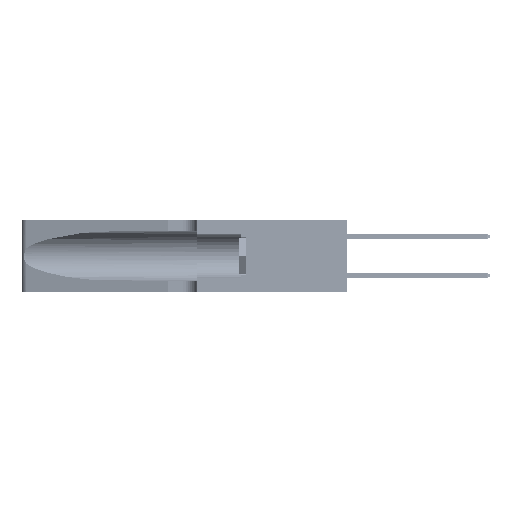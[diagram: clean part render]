
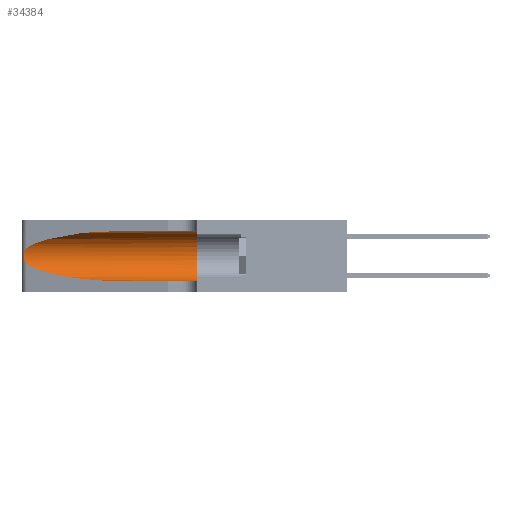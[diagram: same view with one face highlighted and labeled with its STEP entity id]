
A CAD part, left-side view. The second image highlights one B-rep face of the part: STEP entity #34384.
In plain terms, the highlighted cylindrical face has radius 3.308 mm (diameter 6.617 mm), a partial arc.
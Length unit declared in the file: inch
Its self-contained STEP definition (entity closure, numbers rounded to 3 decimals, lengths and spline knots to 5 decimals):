
#969 = VERTEX_POINT ( 'NONE', #30468 ) ;
#2251 = EDGE_CURVE ( 'NONE', #35612, #40799, #40156, .T. ) ;
#2321 = VECTOR ( 'NONE', #39115, 39.37008 ) ;
#2410 = CARTESIAN_POINT ( 'NONE',  ( 0.25555, 1.22993, 0.14849 ) ) ;
#3430 = EDGE_LOOP ( 'NONE', ( #4043, #3513, #14222, #49660, #28067, #21166 ) ) ;
#3513 = ORIENTED_EDGE ( 'NONE', *, *, #25475, .T. ) ;
#3804 = CARTESIAN_POINT ( 'NONE',  ( 0.1305, 1.61858, 0.185 ) ) ;
#3855 =( BOUNDED_CURVE ( )  B_SPLINE_CURVE ( 3, ( #22449, #6502, #34517, #10548 ),
 .UNSPECIFIED., .F., .F. ) 
 B_SPLINE_CURVE_WITH_KNOTS ( ( 4, 4 ),
 ( 3.44316, 4.71239 ),
 .UNSPECIFIED. ) 
 CURVE ( )  GEOMETRIC_REPRESENTATION_ITEM ( )  RATIONAL_B_SPLINE_CURVE ( ( 1., 0.87, 0.87, 1. ) ) 
 REPRESENTATION_ITEM ( '' )  );
#4043 = ORIENTED_EDGE ( 'NONE', *, *, #20420, .T. ) ;
#4616 = AXIS2_PLACEMENT_3D ( 'NONE', #23499, #51512, #27527 ) ;
#5135 = CARTESIAN_POINT ( 'NONE',  ( 0.1305, 1.61858, 0.05475 ) ) ;
#5563 = AXIS2_PLACEMENT_3D ( 'NONE', #3804, #27838, #27506 ) ;
#6502 = CARTESIAN_POINT ( 'NONE',  ( 0.2373, 1.15595, 0.08982 ) ) ;
#7084 = CARTESIAN_POINT ( 'NONE',  ( 0.18966, 0.96281, 0.31525 ) ) ;
#8003 = EDGE_CURVE ( 'NONE', #33133, #19246, #3855, .T. ) ;
#9632 = CARTESIAN_POINT ( 'NONE',  ( 0.25487, 1.22718, 0.22369 ) ) ;
#10352 = CARTESIAN_POINT ( 'NONE',  ( 0.25787, 1.23484, 0.2124 ) ) ;
#10548 = CARTESIAN_POINT ( 'NONE',  ( 0.1305, 0.72297, 0.05475 ) ) ;
#13043 = LINE ( 'NONE', #47167, #2321 ) ;
#13933 = B_SPLINE_CURVE_WITH_KNOTS ( 'NONE', 3,
 ( #26298, #38174, #34328, #10352, #38343, #14393, #42364, #18399, #46371, #22433, #50443, #26474, #2410, #30467 ),
 .UNSPECIFIED., .F., .F.,
 ( 4, 2, 2, 2, 2, 2, 4 ),
 ( 0., 0.00027, 0.00053, 0.00107, 0.0016, 0.00187, 0.00214 ),
 .UNSPECIFIED. ) ;
#14222 = ORIENTED_EDGE ( 'NONE', *, *, #8003, .T. ) ;
#14393 = CARTESIAN_POINT ( 'NONE',  ( 0.26018, 1.23835, 0.19895 ) ) ;
#15142 = CARTESIAN_POINT ( 'NONE',  ( 0.25487, 1.22718, 0.22369 ) ) ;
#18047 = FACE_OUTER_BOUND ( 'NONE', #3430, .T. ) ;
#18399 = CARTESIAN_POINT ( 'NONE',  ( 0.26075, 1.23896, 0.178 ) ) ;
#18468 = VECTOR ( 'NONE', #29140, 39.37008 ) ;
#19246 = VERTEX_POINT ( 'NONE', #25216 ) ;
#20420 = EDGE_CURVE ( 'NONE', #969, #38489, #44287, .T. ) ;
#21166 = ORIENTED_EDGE ( 'NONE', *, *, #46929, .F. ) ;
#22433 = CARTESIAN_POINT ( 'NONE',  ( 0.25856, 1.23593, 0.16098 ) ) ;
#22449 = CARTESIAN_POINT ( 'NONE',  ( 0.25487, 1.22718, 0.14631 ) ) ;
#23019 = CARTESIAN_POINT ( 'NONE',  ( 0.1305, 0.72297, 0.31525 ) ) ;
#23499 = CARTESIAN_POINT ( 'NONE',  ( 0.1305, 0.35, 0.185 ) ) ;
#23575 = CARTESIAN_POINT ( 'NONE',  ( 0.25487, 1.22718, 0.14631 ) ) ;
#25216 = CARTESIAN_POINT ( 'NONE',  ( 0.1305, 0.72297, 0.05475 ) ) ;
#25475 = EDGE_CURVE ( 'NONE', #38489, #33133, #13933, .T. ) ;
#26107 = EDGE_CURVE ( 'NONE', #19246, #40799, #50428, .T. ) ;
#26298 = CARTESIAN_POINT ( 'NONE',  ( 0.25487, 1.22718, 0.22369 ) ) ;
#26474 = CARTESIAN_POINT ( 'NONE',  ( 0.25639, 1.23186, 0.15144 ) ) ;
#27506 = DIRECTION ( 'NONE',  ( 0., 0., -1. ) ) ;
#27527 = DIRECTION ( 'NONE',  ( 0., 0., 1. ) ) ;
#27838 = DIRECTION ( 'NONE',  ( 0., -1., 0. ) ) ;
#27983 = CARTESIAN_POINT ( 'NONE',  ( 0.1305, 0.35, 0.05475 ) ) ;
#28067 = ORIENTED_EDGE ( 'NONE', *, *, #2251, .F. ) ;
#29140 = DIRECTION ( 'NONE',  ( 0., -1., 0. ) ) ;
#30467 = CARTESIAN_POINT ( 'NONE',  ( 0.25487, 1.22718, 0.14631 ) ) ;
#30468 = CARTESIAN_POINT ( 'NONE',  ( 0.1305, 0.72297, 0.31525 ) ) ;
#33133 = VERTEX_POINT ( 'NONE', #23575 ) ;
#34328 = CARTESIAN_POINT ( 'NONE',  ( 0.25639, 1.23184, 0.21858 ) ) ;
#34384 = ADVANCED_FACE ( 'NONE', ( #18047 ), #46175, .F. ) ;
#34517 = CARTESIAN_POINT ( 'NONE',  ( 0.18966, 0.96281, 0.05475 ) ) ;
#35612 = VERTEX_POINT ( 'NONE', #47216 ) ;
#38174 = CARTESIAN_POINT ( 'NONE',  ( 0.25555, 1.22994, 0.2215 ) ) ;
#38343 = CARTESIAN_POINT ( 'NONE',  ( 0.25854, 1.2359, 0.20912 ) ) ;
#38489 = VERTEX_POINT ( 'NONE', #9632 ) ;
#39099 = CARTESIAN_POINT ( 'NONE',  ( 0.2373, 1.15595, 0.28018 ) ) ;
#39115 = DIRECTION ( 'NONE',  ( 0., -1., 0. ) ) ;
#40156 = CIRCLE ( 'NONE', #4616, 0.13025 ) ;
#40799 = VERTEX_POINT ( 'NONE', #27983 ) ;
#42364 = CARTESIAN_POINT ( 'NONE',  ( 0.26075, 1.23896, 0.19203 ) ) ;
#44287 =( BOUNDED_CURVE ( )  B_SPLINE_CURVE ( 3, ( #23019, #7084, #39099, #15142 ),
 .UNSPECIFIED., .F., .F. ) 
 B_SPLINE_CURVE_WITH_KNOTS ( ( 4, 4 ),
 ( 1.5708, 2.84003 ),
 .UNSPECIFIED. ) 
 CURVE ( )  GEOMETRIC_REPRESENTATION_ITEM ( )  RATIONAL_B_SPLINE_CURVE ( ( 1., 0.87, 0.87, 1. ) ) 
 REPRESENTATION_ITEM ( '' )  );
#46175 = CYLINDRICAL_SURFACE ( 'NONE', #5563, 0.13025 ) ;
#46371 = CARTESIAN_POINT ( 'NONE',  ( 0.26017, 1.23833, 0.17102 ) ) ;
#46929 = EDGE_CURVE ( 'NONE', #969, #35612, #13043, .T. ) ;
#47167 = CARTESIAN_POINT ( 'NONE',  ( 0.1305, 1.61858, 0.31525 ) ) ;
#47216 = CARTESIAN_POINT ( 'NONE',  ( 0.1305, 0.35, 0.31525 ) ) ;
#49660 = ORIENTED_EDGE ( 'NONE', *, *, #26107, .T. ) ;
#50428 = LINE ( 'NONE', #5135, #18468 ) ;
#50443 = CARTESIAN_POINT ( 'NONE',  ( 0.25789, 1.23486, 0.15765 ) ) ;
#51512 = DIRECTION ( 'NONE',  ( 0., 1., 0. ) ) ;
